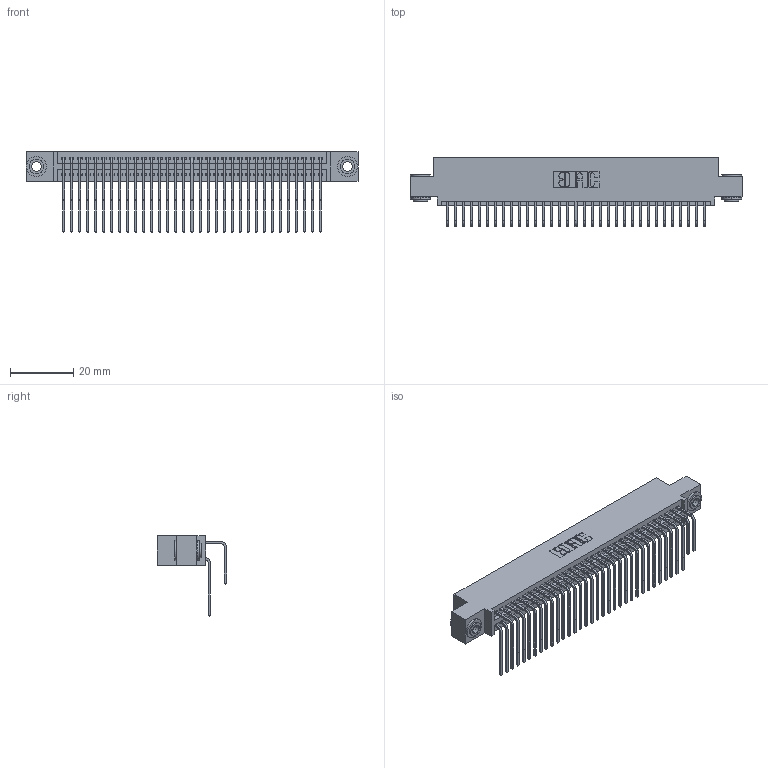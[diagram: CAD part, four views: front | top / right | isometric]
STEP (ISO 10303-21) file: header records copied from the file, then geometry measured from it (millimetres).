
FILE_DESCRIPTION (( 'STEP AP203' ), '1' );
FILE_NAME ('395-066-558-503.STEP', '2018-11-25T06:15:52', ( '' ), ( '' ), 'SwSTEP 2.0', 'SolidWorks 2016', '' );
FILE_SCHEMA (( 'CONFIG_CONTROL_DESIGN' ));
Length unit declared in the file: inch
Products named in the file (5): 345-292-001_558 Tail - 2; 345 Part_0.110 Offset - 0.156 Dia-TH; 345-292-001_558 559 Tail - 1; 345-250-002_345-250-002-102; 395-066-558-503
Assembly tree (69 placements, depth 2):
  395-066-558-503
    345 Part_0.110 Offset - 0.156 Dia-TH
    345-292-001_558 559 Tail - 1  x33
    345-292-001_558 Tail - 2  x33
    345-250-002_345-250-002-102  x2
Bounding box: 105.03 x 21.83 x 25.53 mm (x, y, z)
Volume: 10445.8 mm3; surface area: 17354.5 mm2
Topology: 69 solids, 69 shells, 3600 faces, 10659 edges, 7014 vertices
Faces by surface type: plane 2404, cylinder 1188, cone 8
Entity records: 29538 total; most frequent: CARTESIAN_POINT 4982, ORIENTED_EDGE 4858, DIRECTION 4407, EDGE_CURVE 2429, VECTOR 2101, LINE 2101, VERTEX_POINT 1614, AXIS2_PLACEMENT_3D 1153
